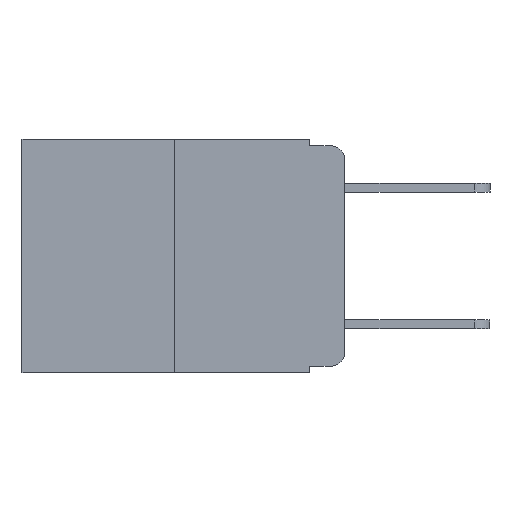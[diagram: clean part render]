
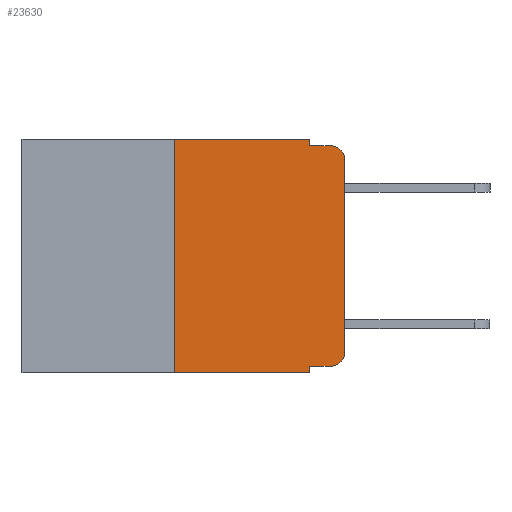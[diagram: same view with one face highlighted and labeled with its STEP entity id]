
A CAD part, left-side view. The second image highlights one B-rep face of the part: STEP entity #23630.
In plain terms, the highlighted planar face has unit normal (-1, 0, 0).
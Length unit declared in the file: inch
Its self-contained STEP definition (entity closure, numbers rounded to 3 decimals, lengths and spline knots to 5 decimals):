
#130 = LINE ( 'NONE', #3485, #9591 ) ;
#208 = CARTESIAN_POINT ( 'NONE',  ( 0., 0.051, 0. ) ) ;
#380 = EDGE_CURVE ( 'NONE', #15830, #10126, #16804, .T. ) ;
#624 = LINE ( 'NONE', #1847, #19762 ) ;
#667 = DIRECTION ( 'NONE',  ( 0., 0., 1. ) ) ;
#710 = CARTESIAN_POINT ( 'NONE',  ( 0., 0., 0. ) ) ;
#764 = FACE_OUTER_BOUND ( 'NONE', #11885, .T. ) ;
#815 = CIRCLE ( 'NONE', #11707, 0.02 ) ;
#1310 = AXIS2_PLACEMENT_3D ( 'NONE', #6754, #19467, #8569 ) ;
#1750 = DIRECTION ( 'NONE',  ( 0., -1., 0. ) ) ;
#1804 = LINE ( 'NONE', #19669, #16035 ) ;
#1847 = CARTESIAN_POINT ( 'NONE',  ( 0., 0.051, -0.333 ) ) ;
#2509 = LINE ( 'NONE', #4804, #20932 ) ;
#3485 = CARTESIAN_POINT ( 'NONE',  ( 0., 0.051, -0.01 ) ) ;
#3775 = CARTESIAN_POINT ( 'NONE',  ( 0., 0.473, -0.343 ) ) ;
#3956 = CARTESIAN_POINT ( 'NONE',  ( 0., 0.02, -0.333 ) ) ;
#4004 = EDGE_CURVE ( 'NONE', #7366, #13964, #130, .T. ) ;
#4060 = CARTESIAN_POINT ( 'NONE',  ( 0., 0.02, -0.313 ) ) ;
#4541 = DIRECTION ( 'NONE',  ( 0., 0., -1. ) ) ;
#4612 = CARTESIAN_POINT ( 'NONE',  ( 0., 0.051, -0.343 ) ) ;
#4804 = CARTESIAN_POINT ( 'NONE',  ( 0., 0.473, 0. ) ) ;
#5074 = VERTEX_POINT ( 'NONE', #10812 ) ;
#5166 = VERTEX_POINT ( 'NONE', #4612 ) ;
#5169 = CARTESIAN_POINT ( 'NONE',  ( 0., 0.25, -0.343 ) ) ;
#5395 = AXIS2_PLACEMENT_3D ( 'NONE', #18367, #20158, #9263 ) ;
#5771 = EDGE_CURVE ( 'NONE', #5074, #15611, #624, .T. ) ;
#5964 = DIRECTION ( 'NONE',  ( 0., 0., -1. ) ) ;
#6428 = CARTESIAN_POINT ( 'NONE',  ( 0., 0.051, 0. ) ) ;
#6744 = LINE ( 'NONE', #6428, #20660 ) ;
#6754 = CARTESIAN_POINT ( 'NONE',  ( 0., 0.02, -0.03 ) ) ;
#7366 = VERTEX_POINT ( 'NONE', #19906 ) ;
#7456 = PLANE ( 'NONE',  #5395 ) ;
#7499 = EDGE_CURVE ( 'NONE', #10327, #5166, #13186, .T. ) ;
#8569 = DIRECTION ( 'NONE',  ( 0., 0., -1. ) ) ;
#9263 = DIRECTION ( 'NONE',  ( 0., 0., -1. ) ) ;
#9591 = VECTOR ( 'NONE', #16026, 39.37008 ) ;
#9625 = DIRECTION ( 'NONE',  ( 0., -1., 0. ) ) ;
#10126 = VERTEX_POINT ( 'NONE', #22702 ) ;
#10327 = VERTEX_POINT ( 'NONE', #5169 ) ;
#10812 = CARTESIAN_POINT ( 'NONE',  ( 0., 0.051, -0.333 ) ) ;
#11176 = VECTOR ( 'NONE', #13358, 39.37008 ) ;
#11224 = CARTESIAN_POINT ( 'NONE',  ( 0., 0.02, -0.01 ) ) ;
#11356 = VECTOR ( 'NONE', #667, 39.37008 ) ;
#11438 = EDGE_CURVE ( 'NONE', #21795, #12193, #2509, .T. ) ;
#11511 = CARTESIAN_POINT ( 'NONE',  ( 0., 0.051, 0. ) ) ;
#11707 = AXIS2_PLACEMENT_3D ( 'NONE', #4060, #16932, #5964 ) ;
#11885 = EDGE_LOOP ( 'NONE', ( #13104, #13215, #13238, #13354, #13495, #13707, #13803, #13921, #14430, #15218 ) ) ;
#12039 = EDGE_CURVE ( 'NONE', #10126, #13964, #14376, .T. ) ;
#12193 = VERTEX_POINT ( 'NONE', #208 ) ;
#12841 = EDGE_CURVE ( 'NONE', #12193, #7366, #20861, .T. ) ;
#13104 = ORIENTED_EDGE ( 'NONE', *, *, #380, .T. ) ;
#13186 = LINE ( 'NONE', #3775, #18594 ) ;
#13215 = ORIENTED_EDGE ( 'NONE', *, *, #12039, .T. ) ;
#13238 = ORIENTED_EDGE ( 'NONE', *, *, #4004, .F. ) ;
#13354 = ORIENTED_EDGE ( 'NONE', *, *, #12841, .F. ) ;
#13358 = DIRECTION ( 'NONE',  ( 0., 0., -1. ) ) ;
#13495 = ORIENTED_EDGE ( 'NONE', *, *, #11438, .F. ) ;
#13707 = ORIENTED_EDGE ( 'NONE', *, *, #19094, .F. ) ;
#13803 = ORIENTED_EDGE ( 'NONE', *, *, #7499, .T. ) ;
#13921 = ORIENTED_EDGE ( 'NONE', *, *, #16495, .F. ) ;
#13964 = VERTEX_POINT ( 'NONE', #11224 ) ;
#14271 = DIRECTION ( 'NONE',  ( 0., 0., 1. ) ) ;
#14376 = CIRCLE ( 'NONE', #1310, 0.02 ) ;
#14430 = ORIENTED_EDGE ( 'NONE', *, *, #5771, .T. ) ;
#15110 = EDGE_CURVE ( 'NONE', #15611, #15830, #815, .T. ) ;
#15218 = ORIENTED_EDGE ( 'NONE', *, *, #15110, .T. ) ;
#15611 = VERTEX_POINT ( 'NONE', #3956 ) ;
#15830 = VERTEX_POINT ( 'NONE', #17386 ) ;
#16026 = DIRECTION ( 'NONE',  ( 0., -1., 0. ) ) ;
#16035 = VECTOR ( 'NONE', #14271, 39.37008 ) ;
#16495 = EDGE_CURVE ( 'NONE', #5074, #5166, #6744, .T. ) ;
#16774 = CARTESIAN_POINT ( 'NONE',  ( 0., 0.25, 0. ) ) ;
#16804 = LINE ( 'NONE', #710, #11356 ) ;
#16932 = DIRECTION ( 'NONE',  ( -1., 0., 0. ) ) ;
#17386 = CARTESIAN_POINT ( 'NONE',  ( 0., 0., -0.313 ) ) ;
#18367 = CARTESIAN_POINT ( 'NONE',  ( 0., 0.473, 0. ) ) ;
#18594 = VECTOR ( 'NONE', #1750, 39.37008 ) ;
#19094 = EDGE_CURVE ( 'NONE', #10327, #21795, #1804, .T. ) ;
#19467 = DIRECTION ( 'NONE',  ( -1., 0., 0. ) ) ;
#19669 = CARTESIAN_POINT ( 'NONE',  ( 0., 0.25, 0. ) ) ;
#19762 = VECTOR ( 'NONE', #9625, 39.37008 ) ;
#19906 = CARTESIAN_POINT ( 'NONE',  ( 0., 0.051, -0.01 ) ) ;
#20158 = DIRECTION ( 'NONE',  ( 1., 0., 0. ) ) ;
#20660 = VECTOR ( 'NONE', #4541, 39.37008 ) ;
#20861 = LINE ( 'NONE', #11511, #11176 ) ;
#20932 = VECTOR ( 'NONE', #23047, 39.37008 ) ;
#21795 = VERTEX_POINT ( 'NONE', #16774 ) ;
#22702 = CARTESIAN_POINT ( 'NONE',  ( 0., 0., -0.03 ) ) ;
#23047 = DIRECTION ( 'NONE',  ( 0., -1., 0. ) ) ;
#23630 = ADVANCED_FACE ( 'NONE', ( #764 ), #7456, .F. ) ;
